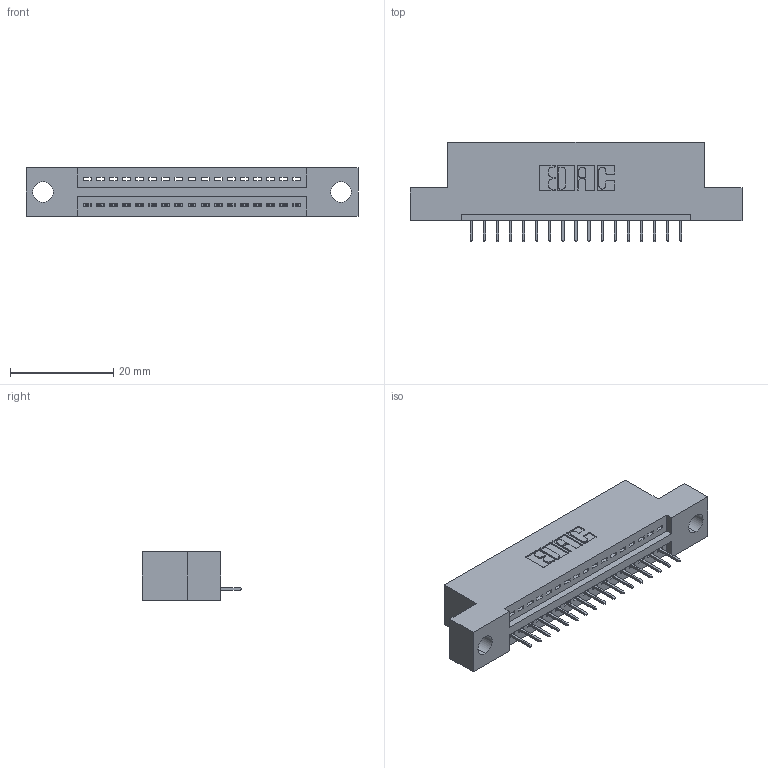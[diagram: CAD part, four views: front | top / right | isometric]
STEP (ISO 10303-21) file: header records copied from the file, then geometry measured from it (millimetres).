
FILE_DESCRIPTION (( 'STEP AP203' ), '1' );
FILE_NAME ('395-017-524-104.STEP', '2021-05-31T14:24:28', ( '' ), ( '' ), 'SwSTEP 2.0', 'SolidWorks 2020', '' );
FILE_SCHEMA (( 'CONFIG_CONTROL_DESIGN' ));
Length unit declared in the file: inch
Products named in the file (3): 345-292-001_345-293-124; 345 Part_Flush Mounting Lugs - 0.156 Dia-TI; 395-017-524-104
Assembly tree (18 placements, depth 2):
  395-017-524-104
    345 Part_Flush Mounting Lugs - 0.156 Dia-TI
    345-292-001_345-293-124  x17
Bounding box: 64.39 x 19.35 x 9.4 mm (x, y, z)
Volume: 5737.8 mm3; surface area: 6913 mm2
Topology: 18 solids, 18 shells, 1194 faces, 3437 edges, 2222 vertices
Faces by surface type: plane 876, cylinder 318
Entity records: 16653 total; most frequent: CARTESIAN_POINT 2893, ORIENTED_EDGE 2842, DIRECTION 2563, EDGE_CURVE 1421, LINE 1225, VECTOR 1225, VERTEX_POINT 942, AXIS2_PLACEMENT_3D 669
